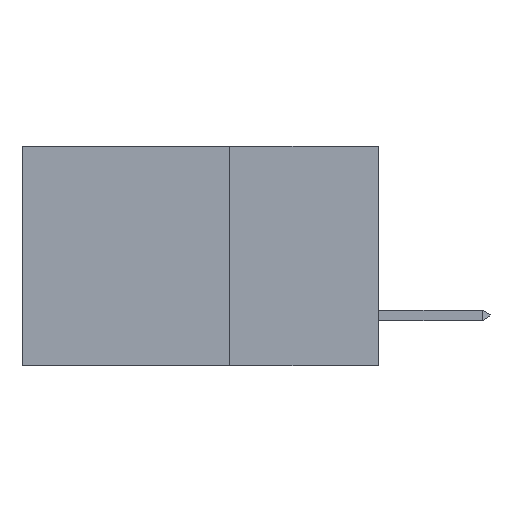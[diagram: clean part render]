
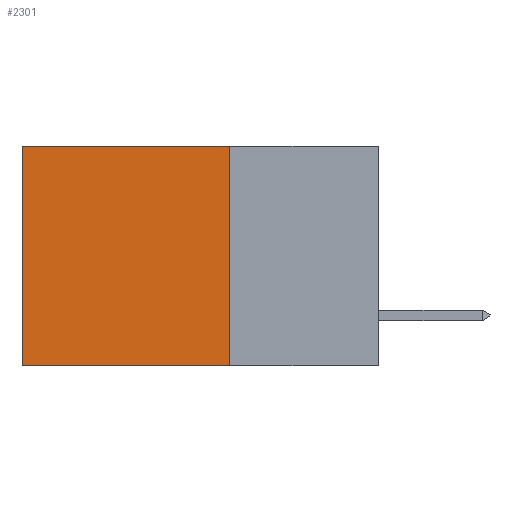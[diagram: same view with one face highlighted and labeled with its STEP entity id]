
A CAD part, left-side view. The second image highlights one B-rep face of the part: STEP entity #2301.
In plain terms, the highlighted planar face has unit normal (-1, 0, 0).
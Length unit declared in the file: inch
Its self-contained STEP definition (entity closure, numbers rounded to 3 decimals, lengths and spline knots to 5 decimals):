
#433 = CARTESIAN_POINT ( 'NONE',  ( 0.2615, 0.25, 0. ) ) ;
#1159 = VERTEX_POINT ( 'NONE', #14243 ) ;
#2301 = ADVANCED_FACE ( 'NONE', ( #13955 ), #6835, .F. ) ;
#2425 = DIRECTION ( 'NONE',  ( 1., 0., 0. ) ) ;
#2589 = LINE ( 'NONE', #11895, #11789 ) ;
#3287 = LINE ( 'NONE', #4098, #11026 ) ;
#3330 = EDGE_CURVE ( 'NONE', #4120, #5723, #2589, .T. ) ;
#4098 = CARTESIAN_POINT ( 'NONE',  ( 0.2615, 0.25, 0. ) ) ;
#4120 = VERTEX_POINT ( 'NONE', #433 ) ;
#5543 = DIRECTION ( 'NONE',  ( 0., 1., 0. ) ) ;
#5723 = VERTEX_POINT ( 'NONE', #10473 ) ;
#5735 = EDGE_CURVE ( 'NONE', #1159, #11800, #10767, .T. ) ;
#6023 = DIRECTION ( 'NONE',  ( 0., 0., -1. ) ) ;
#6835 = PLANE ( 'NONE',  #10327 ) ;
#7127 = DIRECTION ( 'NONE',  ( 0., 0., -1. ) ) ;
#7478 = EDGE_LOOP ( 'NONE', ( #11654, #10849, #13543, #8291 ) ) ;
#7517 = EDGE_CURVE ( 'NONE', #5723, #11800, #8367, .T. ) ;
#8291 = ORIENTED_EDGE ( 'NONE', *, *, #9325, .T. ) ;
#8296 = CARTESIAN_POINT ( 'NONE',  ( 0.2615, 0.25, -0.37 ) ) ;
#8367 = LINE ( 'NONE', #8296, #11714 ) ;
#8484 = CARTESIAN_POINT ( 'NONE',  ( 0.2615, 0.6, -0.37 ) ) ;
#9325 = EDGE_CURVE ( 'NONE', #4120, #1159, #3287, .T. ) ;
#10327 = AXIS2_PLACEMENT_3D ( 'NONE', #12639, #2425, #11379 ) ;
#10473 = CARTESIAN_POINT ( 'NONE',  ( 0.2615, 0.25, -0.37 ) ) ;
#10584 = DIRECTION ( 'NONE',  ( 0., 1., 0. ) ) ;
#10767 = LINE ( 'NONE', #8484, #13885 ) ;
#10849 = ORIENTED_EDGE ( 'NONE', *, *, #7517, .F. ) ;
#11026 = VECTOR ( 'NONE', #5543, 39.37008 ) ;
#11254 = CARTESIAN_POINT ( 'NONE',  ( 0.2615, 0.6, -0.37 ) ) ;
#11379 = DIRECTION ( 'NONE',  ( 0., 0., -1. ) ) ;
#11654 = ORIENTED_EDGE ( 'NONE', *, *, #5735, .T. ) ;
#11714 = VECTOR ( 'NONE', #10584, 39.37008 ) ;
#11789 = VECTOR ( 'NONE', #7127, 39.37008 ) ;
#11800 = VERTEX_POINT ( 'NONE', #11254 ) ;
#11895 = CARTESIAN_POINT ( 'NONE',  ( 0.2615, 0.25, -0.37 ) ) ;
#12639 = CARTESIAN_POINT ( 'NONE',  ( 0.2615, 0.25, -0.37 ) ) ;
#13543 = ORIENTED_EDGE ( 'NONE', *, *, #3330, .F. ) ;
#13885 = VECTOR ( 'NONE', #6023, 39.37008 ) ;
#13955 = FACE_OUTER_BOUND ( 'NONE', #7478, .T. ) ;
#14243 = CARTESIAN_POINT ( 'NONE',  ( 0.2615, 0.6, 0. ) ) ;
